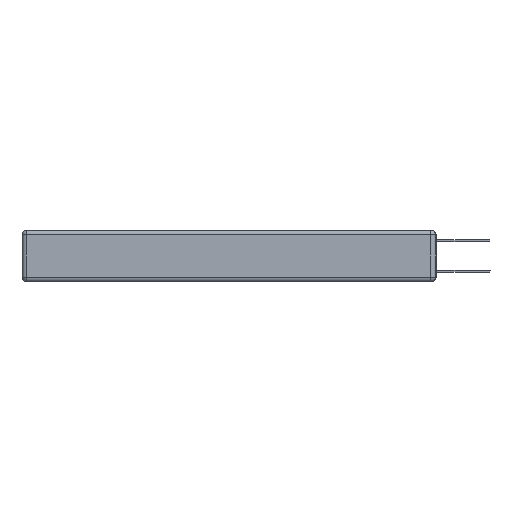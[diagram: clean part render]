
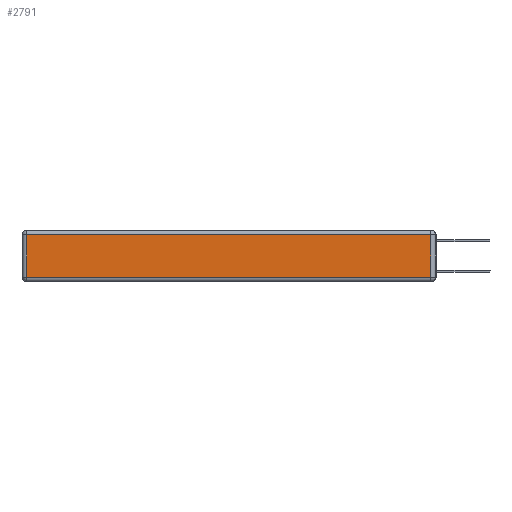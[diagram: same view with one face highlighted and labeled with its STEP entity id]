
A CAD part, left-side view. The second image highlights one B-rep face of the part: STEP entity #2791.
In plain terms, the highlighted planar face has unit normal (-1, 0, 0).
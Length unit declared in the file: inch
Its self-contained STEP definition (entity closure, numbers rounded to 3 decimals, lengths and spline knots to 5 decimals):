
#1457 = ORIENTED_EDGE ( 'NONE', *, *, #6154, .T. ) ;
#1805 = EDGE_CURVE ( 'NONE', #13236, #15845, #12661, .T. ) ;
#1934 = DIRECTION ( 'NONE',  ( -1., 0., 0. ) ) ;
#1994 = CARTESIAN_POINT ( 'NONE',  ( 0., 0., -0.313 ) ) ;
#2586 = CARTESIAN_POINT ( 'NONE',  ( 0., 2.72, -0.343 ) ) ;
#2791 = ADVANCED_FACE ( 'NONE', ( #13161 ), #4510, .T. ) ;
#2887 = EDGE_CURVE ( 'NONE', #15845, #4873, #13490, .T. ) ;
#2986 = CARTESIAN_POINT ( 'NONE',  ( 0., 2.72, -0.03 ) ) ;
#3162 = DIRECTION ( 'NONE',  ( 0., -1., 0. ) ) ;
#3517 = DIRECTION ( 'NONE',  ( 0., 0., 1. ) ) ;
#4498 = CARTESIAN_POINT ( 'NONE',  ( 0., 0.03, -0.313 ) ) ;
#4510 = PLANE ( 'NONE',  #11985 ) ;
#4873 = VERTEX_POINT ( 'NONE', #2986 ) ;
#4982 = CARTESIAN_POINT ( 'NONE',  ( 0., 2.72, -0.313 ) ) ;
#5721 = LINE ( 'NONE', #1994, #11072 ) ;
#5879 = EDGE_CURVE ( 'NONE', #4873, #13341, #6061, .T. ) ;
#6061 = LINE ( 'NONE', #2586, #12888 ) ;
#6154 = EDGE_CURVE ( 'NONE', #13341, #13236, #5721, .T. ) ;
#6374 = CARTESIAN_POINT ( 'NONE',  ( 0., 0.03, -0.343 ) ) ;
#7039 = ORIENTED_EDGE ( 'NONE', *, *, #5879, .T. ) ;
#7170 = VECTOR ( 'NONE', #13415, 39.37008 ) ;
#8379 = CARTESIAN_POINT ( 'NONE',  ( 0., 2.75, -0.03 ) ) ;
#8544 = DIRECTION ( 'NONE',  ( 0., 0., -1. ) ) ;
#8617 = ORIENTED_EDGE ( 'NONE', *, *, #2887, .T. ) ;
#8938 = ORIENTED_EDGE ( 'NONE', *, *, #1805, .T. ) ;
#10108 = CARTESIAN_POINT ( 'NONE',  ( 0., 0.03, -0.03 ) ) ;
#10998 = EDGE_LOOP ( 'NONE', ( #1457, #8938, #8617, #7039 ) ) ;
#11072 = VECTOR ( 'NONE', #3162, 39.37008 ) ;
#11985 = AXIS2_PLACEMENT_3D ( 'NONE', #15913, #1934, #3517 ) ;
#12638 = VECTOR ( 'NONE', #15395, 39.37008 ) ;
#12661 = LINE ( 'NONE', #6374, #12638 ) ;
#12888 = VECTOR ( 'NONE', #8544, 39.37008 ) ;
#13161 = FACE_OUTER_BOUND ( 'NONE', #10998, .T. ) ;
#13236 = VERTEX_POINT ( 'NONE', #4498 ) ;
#13341 = VERTEX_POINT ( 'NONE', #4982 ) ;
#13415 = DIRECTION ( 'NONE',  ( 0., 1., 0. ) ) ;
#13490 = LINE ( 'NONE', #8379, #7170 ) ;
#15395 = DIRECTION ( 'NONE',  ( 0., 0., 1. ) ) ;
#15845 = VERTEX_POINT ( 'NONE', #10108 ) ;
#15913 = CARTESIAN_POINT ( 'NONE',  ( 0., 0., -0.343 ) ) ;
